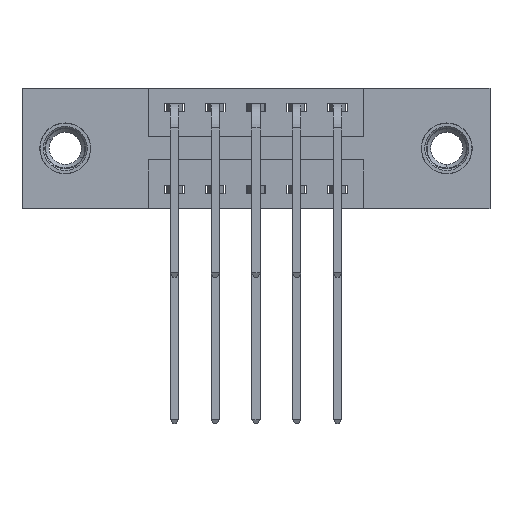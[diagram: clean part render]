
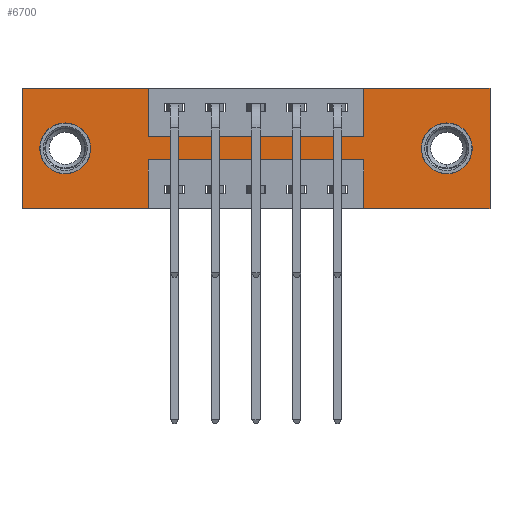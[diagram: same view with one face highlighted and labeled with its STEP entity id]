
A CAD part, front view. The second image highlights one B-rep face of the part: STEP entity #6700.
In plain terms, the highlighted planar face has unit normal (0, -1, 0).
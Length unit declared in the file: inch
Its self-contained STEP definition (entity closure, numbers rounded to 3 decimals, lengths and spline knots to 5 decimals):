
#229 = EDGE_CURVE ( 'NONE', #7666, #9998, #4791, .T. ) ;
#235 = CARTESIAN_POINT ( 'NONE',  ( 0.3875, 0., -0.15 ) ) ;
#385 = DIRECTION ( 'NONE',  ( 0., 0., -1. ) ) ;
#483 = VECTOR ( 'NONE', #5702, 39.37008 ) ;
#552 = EDGE_CURVE ( 'NONE', #6117, #2619, #1971, .T. ) ;
#607 = EDGE_CURVE ( 'NONE', #9230, #7666, #1506, .T. ) ;
#622 = EDGE_CURVE ( 'NONE', #1239, #9230, #2245, .T. ) ;
#654 = EDGE_CURVE ( 'NONE', #5240, #1239, #10583, .T. ) ;
#712 = EDGE_CURVE ( 'NONE', #2821, #8894, #6121, .T. ) ;
#729 = EDGE_CURVE ( 'NONE', #871, #2821, #5847, .T. ) ;
#737 = CARTESIAN_POINT ( 'NONE',  ( 1.3025, 0., -0.263 ) ) ;
#747 = DIRECTION ( 'NONE',  ( 0., 0., -1. ) ) ;
#753 = CARTESIAN_POINT ( 'NONE',  ( 0.3875, 0., 0. ) ) ;
#785 = CARTESIAN_POINT ( 'NONE',  ( 1.435, 0., 0. ) ) ;
#849 = LINE ( 'NONE', #785, #3131 ) ;
#861 = EDGE_CURVE ( 'NONE', #1917, #871, #10537, .T. ) ;
#871 = VERTEX_POINT ( 'NONE', #235 ) ;
#945 = EDGE_CURVE ( 'NONE', #4989, #1917, #4205, .T. ) ;
#1026 = DIRECTION ( 'NONE',  ( 0., 0., -1. ) ) ;
#1053 = PLANE ( 'NONE',  #1160 ) ;
#1089 = CARTESIAN_POINT ( 'NONE',  ( 0., 0., -0.37 ) ) ;
#1118 = DIRECTION ( 'NONE',  ( 0., -1., 0. ) ) ;
#1160 = AXIS2_PLACEMENT_3D ( 'NONE', #1089, #1118, #1026 ) ;
#1239 = VERTEX_POINT ( 'NONE', #9096 ) ;
#1278 = CARTESIAN_POINT ( 'NONE',  ( 0.3875, 0., -0.22 ) ) ;
#1325 = VECTOR ( 'NONE', #385, 39.37008 ) ;
#1506 = LINE ( 'NONE', #5579, #483 ) ;
#1549 = VECTOR ( 'NONE', #3985, 39.37008 ) ;
#1567 = VERTEX_POINT ( 'NONE', #7340 ) ;
#1877 = DIRECTION ( 'NONE',  ( -1., 0., 0. ) ) ;
#1892 = CARTESIAN_POINT ( 'NONE',  ( 0., 0., -0.37 ) ) ;
#1917 = VERTEX_POINT ( 'NONE', #5075 ) ;
#1971 = CIRCLE ( 'NONE', #4294, 0.078 ) ;
#2245 = LINE ( 'NONE', #3369, #3829 ) ;
#2270 = FACE_BOUND ( 'NONE', #10791, .T. ) ;
#2305 = DIRECTION ( 'NONE',  ( 0., 0., 1. ) ) ;
#2322 = LINE ( 'NONE', #4226, #1549 ) ;
#2415 = EDGE_CURVE ( 'NONE', #8630, #5240, #8040, .T. ) ;
#2619 = VERTEX_POINT ( 'NONE', #737 ) ;
#2766 = CARTESIAN_POINT ( 'NONE',  ( 1.0475, 0., 0. ) ) ;
#2821 = VERTEX_POINT ( 'NONE', #6861 ) ;
#2869 = DIRECTION ( 'NONE',  ( 0., 0., 1. ) ) ;
#2884 = DIRECTION ( 'NONE',  ( 0., 1., 0. ) ) ;
#2904 = CARTESIAN_POINT ( 'NONE',  ( 0.1325, 0., -0.185 ) ) ;
#2959 = EDGE_CURVE ( 'NONE', #1567, #9934, #5887, .T. ) ;
#3131 = VECTOR ( 'NONE', #747, 39.37008 ) ;
#3236 = VECTOR ( 'NONE', #10760, 39.37008 ) ;
#3350 = DIRECTION ( 'NONE',  ( -1., 0., 0. ) ) ;
#3369 = CARTESIAN_POINT ( 'NONE',  ( 0.3875, 0., -0.22 ) ) ;
#3448 = DIRECTION ( 'NONE',  ( 0., 0., -1. ) ) ;
#3601 = DIRECTION ( 'NONE',  ( 0., 1., 0. ) ) ;
#3789 = VECTOR ( 'NONE', #10706, 39.37008 ) ;
#3829 = VECTOR ( 'NONE', #3350, 39.37008 ) ;
#3985 = DIRECTION ( 'NONE',  ( 1., 0., 0. ) ) ;
#4099 = CARTESIAN_POINT ( 'NONE',  ( 0., 0., 0. ) ) ;
#4112 = VECTOR ( 'NONE', #8915, 39.37008 ) ;
#4205 = LINE ( 'NONE', #10718, #3236 ) ;
#4226 = CARTESIAN_POINT ( 'NONE',  ( 0., 0., 0. ) ) ;
#4231 = EDGE_CURVE ( 'NONE', #9998, #4989, #5135, .T. ) ;
#4294 = AXIS2_PLACEMENT_3D ( 'NONE', #6417, #3601, #3448 ) ;
#4454 = FACE_BOUND ( 'NONE', #7715, .T. ) ;
#4478 = CARTESIAN_POINT ( 'NONE',  ( 0.1325, 0., -0.263 ) ) ;
#4617 = CARTESIAN_POINT ( 'NONE',  ( 1.0475, 0., 0. ) ) ;
#4723 = VECTOR ( 'NONE', #8921, 39.37008 ) ;
#4791 = LINE ( 'NONE', #8525, #4112 ) ;
#4984 = EDGE_CURVE ( 'NONE', #8894, #7817, #2322, .T. ) ;
#4989 = VERTEX_POINT ( 'NONE', #4099 ) ;
#5075 = CARTESIAN_POINT ( 'NONE',  ( 0.3875, 0., 0. ) ) ;
#5135 = LINE ( 'NONE', #9163, #4723 ) ;
#5240 = VERTEX_POINT ( 'NONE', #11164 ) ;
#5281 = ORIENTED_EDGE ( 'NONE', *, *, #229, .F. ) ;
#5401 = CARTESIAN_POINT ( 'NONE',  ( 0., 0., -0.37 ) ) ;
#5461 = CARTESIAN_POINT ( 'NONE',  ( 1.0475, 0., -0.37 ) ) ;
#5465 = DIRECTION ( 'NONE',  ( 0., 0., 1. ) ) ;
#5495 = CARTESIAN_POINT ( 'NONE',  ( 1.3025, 0., -0.107 ) ) ;
#5579 = CARTESIAN_POINT ( 'NONE',  ( 0.3875, 0., -0.37 ) ) ;
#5588 = VECTOR ( 'NONE', #2305, 39.37008 ) ;
#5702 = DIRECTION ( 'NONE',  ( 0., 0., -1. ) ) ;
#5847 = LINE ( 'NONE', #10632, #3789 ) ;
#5887 = CIRCLE ( 'NONE', #7631, 0.078 ) ;
#6117 = VERTEX_POINT ( 'NONE', #5495 ) ;
#6121 = LINE ( 'NONE', #2766, #5588 ) ;
#6142 = CARTESIAN_POINT ( 'NONE',  ( 1.435, 0., 0. ) ) ;
#6169 = CIRCLE ( 'NONE', #9823, 0.078 ) ;
#6417 = CARTESIAN_POINT ( 'NONE',  ( 1.3025, 0., -0.185 ) ) ;
#6639 = CARTESIAN_POINT ( 'NONE',  ( 1.435, 0., -0.37 ) ) ;
#6700 = ADVANCED_FACE ( 'NONE', ( #2270, #4454, #11051 ), #1053, .T. ) ;
#6861 = CARTESIAN_POINT ( 'NONE',  ( 1.0475, 0., -0.15 ) ) ;
#7228 = CIRCLE ( 'NONE', #11237, 0.078 ) ;
#7340 = CARTESIAN_POINT ( 'NONE',  ( 0.1325, 0., -0.107 ) ) ;
#7631 = AXIS2_PLACEMENT_3D ( 'NONE', #10882, #10851, #10354 ) ;
#7663 = VECTOR ( 'NONE', #1877, 39.37008 ) ;
#7666 = VERTEX_POINT ( 'NONE', #8864 ) ;
#7715 = EDGE_LOOP ( 'NONE', ( #8251, #9062 ) ) ;
#7817 = VERTEX_POINT ( 'NONE', #6142 ) ;
#7828 = DIRECTION ( 'NONE',  ( 0., 0., -1. ) ) ;
#7840 = DIRECTION ( 'NONE',  ( 0., 1., 0. ) ) ;
#7856 = CARTESIAN_POINT ( 'NONE',  ( 1.3025, 0., -0.185 ) ) ;
#7893 = ORIENTED_EDGE ( 'NONE', *, *, #552, .T. ) ;
#8040 = LINE ( 'NONE', #1892, #7663 ) ;
#8072 = ORIENTED_EDGE ( 'NONE', *, *, #4231, .F. ) ;
#8251 = ORIENTED_EDGE ( 'NONE', *, *, #2959, .T. ) ;
#8305 = EDGE_LOOP ( 'NONE', ( #8976, #11070, #9869, #9100, #9921, #9037, #9015, #9080, #8398, #9333, #8072, #5281 ) ) ;
#8398 = ORIENTED_EDGE ( 'NONE', *, *, #861, .F. ) ;
#8410 = EDGE_CURVE ( 'NONE', #2619, #6117, #7228, .T. ) ;
#8525 = CARTESIAN_POINT ( 'NONE',  ( 0., 0., -0.37 ) ) ;
#8630 = VERTEX_POINT ( 'NONE', #6639 ) ;
#8864 = CARTESIAN_POINT ( 'NONE',  ( 0.3875, 0., -0.37 ) ) ;
#8894 = VERTEX_POINT ( 'NONE', #4617 ) ;
#8915 = DIRECTION ( 'NONE',  ( -1., 0., 0. ) ) ;
#8921 = DIRECTION ( 'NONE',  ( 0., 0., 1. ) ) ;
#8976 = ORIENTED_EDGE ( 'NONE', *, *, #607, .F. ) ;
#9015 = ORIENTED_EDGE ( 'NONE', *, *, #712, .F. ) ;
#9037 = ORIENTED_EDGE ( 'NONE', *, *, #4984, .F. ) ;
#9040 = EDGE_CURVE ( 'NONE', #9934, #1567, #6169, .T. ) ;
#9062 = ORIENTED_EDGE ( 'NONE', *, *, #9040, .T. ) ;
#9080 = ORIENTED_EDGE ( 'NONE', *, *, #729, .F. ) ;
#9096 = CARTESIAN_POINT ( 'NONE',  ( 1.0475, 0., -0.22 ) ) ;
#9100 = ORIENTED_EDGE ( 'NONE', *, *, #2415, .F. ) ;
#9163 = CARTESIAN_POINT ( 'NONE',  ( 0., 0., 0. ) ) ;
#9230 = VERTEX_POINT ( 'NONE', #1278 ) ;
#9293 = EDGE_CURVE ( 'NONE', #7817, #8630, #849, .T. ) ;
#9298 = ORIENTED_EDGE ( 'NONE', *, *, #8410, .T. ) ;
#9333 = ORIENTED_EDGE ( 'NONE', *, *, #945, .F. ) ;
#9823 = AXIS2_PLACEMENT_3D ( 'NONE', #2904, #2884, #2869 ) ;
#9869 = ORIENTED_EDGE ( 'NONE', *, *, #654, .F. ) ;
#9921 = ORIENTED_EDGE ( 'NONE', *, *, #9293, .F. ) ;
#9934 = VERTEX_POINT ( 'NONE', #4478 ) ;
#9998 = VERTEX_POINT ( 'NONE', #5401 ) ;
#10200 = VECTOR ( 'NONE', #5465, 39.37008 ) ;
#10354 = DIRECTION ( 'NONE',  ( 0., 0., 1. ) ) ;
#10537 = LINE ( 'NONE', #753, #1325 ) ;
#10583 = LINE ( 'NONE', #5461, #10200 ) ;
#10632 = CARTESIAN_POINT ( 'NONE',  ( 0.3875, 0., -0.15 ) ) ;
#10706 = DIRECTION ( 'NONE',  ( 1., 0., 0. ) ) ;
#10718 = CARTESIAN_POINT ( 'NONE',  ( 0., 0., 0. ) ) ;
#10760 = DIRECTION ( 'NONE',  ( 1., 0., 0. ) ) ;
#10791 = EDGE_LOOP ( 'NONE', ( #7893, #9298 ) ) ;
#10851 = DIRECTION ( 'NONE',  ( 0., 1., 0. ) ) ;
#10882 = CARTESIAN_POINT ( 'NONE',  ( 0.1325, 0., -0.185 ) ) ;
#11051 = FACE_OUTER_BOUND ( 'NONE', #8305, .T. ) ;
#11070 = ORIENTED_EDGE ( 'NONE', *, *, #622, .F. ) ;
#11164 = CARTESIAN_POINT ( 'NONE',  ( 1.0475, 0., -0.37 ) ) ;
#11237 = AXIS2_PLACEMENT_3D ( 'NONE', #7856, #7840, #7828 ) ;
